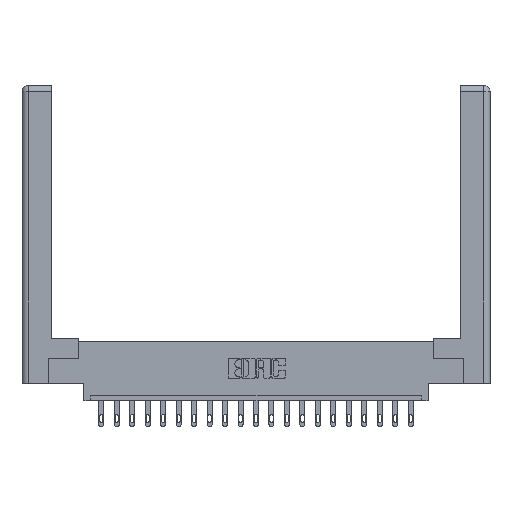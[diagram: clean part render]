
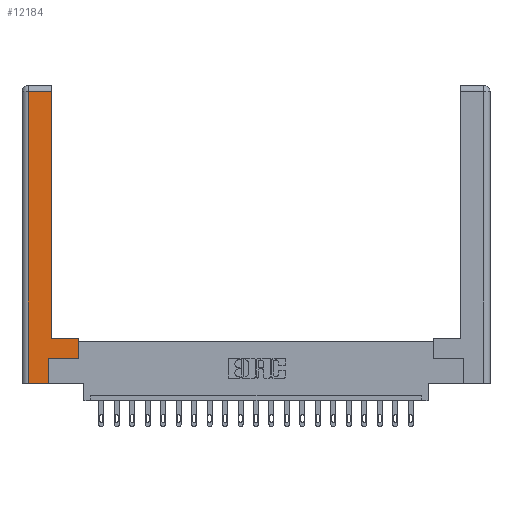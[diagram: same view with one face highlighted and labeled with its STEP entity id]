
A CAD part, top view. The second image highlights one B-rep face of the part: STEP entity #12184.
In plain terms, the highlighted planar face has unit normal (0, 0, 1).
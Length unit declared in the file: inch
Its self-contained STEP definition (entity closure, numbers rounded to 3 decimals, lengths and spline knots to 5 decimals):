
#114 = DIRECTION ( 'NONE',  ( 0., 1., 0. ) ) ;
#298 = ORIENTED_EDGE ( 'NONE', *, *, #4165, .T. ) ;
#382 = LINE ( 'NONE', #8246, #15899 ) ;
#531 = ORIENTED_EDGE ( 'NONE', *, *, #4616, .T. ) ;
#1164 = ORIENTED_EDGE ( 'NONE', *, *, #4594, .T. ) ;
#1265 = VECTOR ( 'NONE', #3855, 39.37008 ) ;
#1272 = FACE_OUTER_BOUND ( 'NONE', #20090, .T. ) ;
#1632 = CARTESIAN_POINT ( 'NONE',  ( 0.565, 0.45, 0. ) ) ;
#1728 = PLANE ( 'NONE',  #5879 ) ;
#2879 = DIRECTION ( 'NONE',  ( -1., 0., 0. ) ) ;
#3006 = CARTESIAN_POINT ( 'NONE',  ( 0.265, 0.245, 0. ) ) ;
#3404 = CARTESIAN_POINT ( 'NONE',  ( 0.565, 0.245, 0. ) ) ;
#3453 = LINE ( 'NONE', #9670, #8535 ) ;
#3570 = VECTOR ( 'NONE', #17845, 39.37008 ) ;
#3747 = DIRECTION ( 'NONE',  ( 1., 0., 0. ) ) ;
#3855 = DIRECTION ( 'NONE',  ( 0., 1., 0. ) ) ;
#3948 = CARTESIAN_POINT ( 'NONE',  ( 0.265, 0., 0. ) ) ;
#4151 = VERTEX_POINT ( 'NONE', #1632 ) ;
#4165 = EDGE_CURVE ( 'NONE', #9062, #4617, #3453, .T. ) ;
#4228 = EDGE_CURVE ( 'NONE', #8321, #4151, #382, .T. ) ;
#4397 = ORIENTED_EDGE ( 'NONE', *, *, #15518, .T. ) ;
#4465 = VERTEX_POINT ( 'NONE', #7193 ) ;
#4594 = EDGE_CURVE ( 'NONE', #4617, #14374, #5702, .T. ) ;
#4616 = EDGE_CURVE ( 'NONE', #14374, #17514, #13615, .T. ) ;
#4617 = VERTEX_POINT ( 'NONE', #16948 ) ;
#5200 = ORIENTED_EDGE ( 'NONE', *, *, #8030, .T. ) ;
#5395 = ORIENTED_EDGE ( 'NONE', *, *, #7913, .T. ) ;
#5574 = DIRECTION ( 'NONE',  ( 0., 1., 0. ) ) ;
#5702 = LINE ( 'NONE', #3948, #17395 ) ;
#5879 = AXIS2_PLACEMENT_3D ( 'NONE', #5883, #6018, #7519 ) ;
#5883 = CARTESIAN_POINT ( 'NONE',  ( 0., 0., 0. ) ) ;
#6018 = DIRECTION ( 'NONE',  ( 0., 0., -1. ) ) ;
#6094 = CARTESIAN_POINT ( 'NONE',  ( 0.565, 0.245, 0. ) ) ;
#6604 = DIRECTION ( 'NONE',  ( 0., -1., 0. ) ) ;
#6626 = CARTESIAN_POINT ( 'NONE',  ( 0.295, 0.45, 0. ) ) ;
#6742 = VECTOR ( 'NONE', #2879, 39.37008 ) ;
#6973 = LINE ( 'NONE', #6094, #19415 ) ;
#7193 = CARTESIAN_POINT ( 'NONE',  ( 0.295, 0.45, 0. ) ) ;
#7519 = DIRECTION ( 'NONE',  ( -1., 0., 0. ) ) ;
#7913 = EDGE_CURVE ( 'NONE', #4151, #4465, #19567, .T. ) ;
#8030 = EDGE_CURVE ( 'NONE', #4465, #16461, #11445, .T. ) ;
#8246 = CARTESIAN_POINT ( 'NONE',  ( 0.565, 0.45, 0. ) ) ;
#8321 = VERTEX_POINT ( 'NONE', #3404 ) ;
#8535 = VECTOR ( 'NONE', #6604, 39.37008 ) ;
#8538 = LINE ( 'NONE', #11130, #6742 ) ;
#8782 = VECTOR ( 'NONE', #5574, 39.37008 ) ;
#9062 = VERTEX_POINT ( 'NONE', #18568 ) ;
#9670 = CARTESIAN_POINT ( 'NONE',  ( 0.0615, 0., 0. ) ) ;
#9987 = ORIENTED_EDGE ( 'NONE', *, *, #4228, .T. ) ;
#11130 = CARTESIAN_POINT ( 'NONE',  ( 0.0615, 2.94, 0. ) ) ;
#11445 = LINE ( 'NONE', #11757, #1265 ) ;
#11757 = CARTESIAN_POINT ( 'NONE',  ( 0.295, 3., 0. ) ) ;
#12184 = ADVANCED_FACE ( 'NONE', ( #1272 ), #1728, .F. ) ;
#13615 = LINE ( 'NONE', #15334, #8782 ) ;
#13819 = CARTESIAN_POINT ( 'NONE',  ( 0.295, 2.94, 0. ) ) ;
#14374 = VERTEX_POINT ( 'NONE', #15681 ) ;
#14997 = EDGE_CURVE ( 'NONE', #16461, #9062, #8538, .T. ) ;
#15334 = CARTESIAN_POINT ( 'NONE',  ( 0.265, 0.245, 0. ) ) ;
#15518 = EDGE_CURVE ( 'NONE', #17514, #8321, #6973, .T. ) ;
#15681 = CARTESIAN_POINT ( 'NONE',  ( 0.265, 0., 0. ) ) ;
#15899 = VECTOR ( 'NONE', #114, 39.37008 ) ;
#16461 = VERTEX_POINT ( 'NONE', #13819 ) ;
#16948 = CARTESIAN_POINT ( 'NONE',  ( 0.0615, 0., 0. ) ) ;
#17185 = DIRECTION ( 'NONE',  ( 1., 0., 0. ) ) ;
#17395 = VECTOR ( 'NONE', #3747, 39.37008 ) ;
#17514 = VERTEX_POINT ( 'NONE', #3006 ) ;
#17845 = DIRECTION ( 'NONE',  ( -1., 0., 0. ) ) ;
#18568 = CARTESIAN_POINT ( 'NONE',  ( 0.0615, 2.94, 0. ) ) ;
#19415 = VECTOR ( 'NONE', #17185, 39.37008 ) ;
#19567 = LINE ( 'NONE', #6626, #3570 ) ;
#20090 = EDGE_LOOP ( 'NONE', ( #5200, #20467, #298, #1164, #531, #4397, #9987, #5395 ) ) ;
#20467 = ORIENTED_EDGE ( 'NONE', *, *, #14997, .T. ) ;
